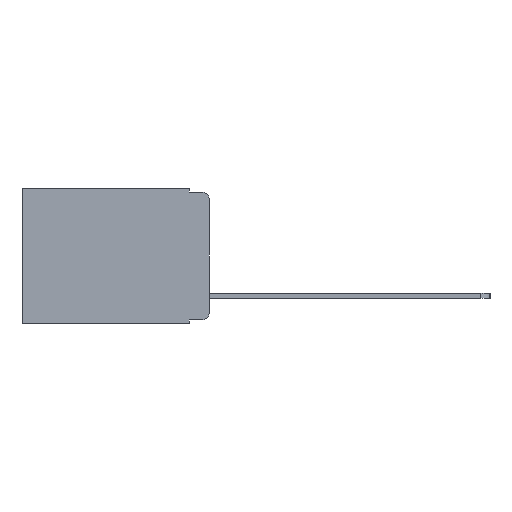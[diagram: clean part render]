
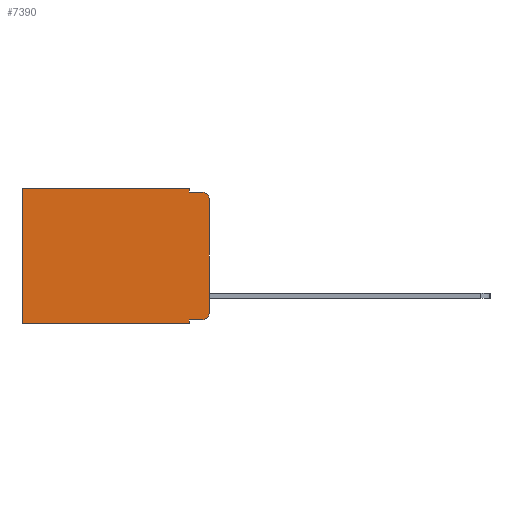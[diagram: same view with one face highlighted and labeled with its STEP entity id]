
A CAD part, left-side view. The second image highlights one B-rep face of the part: STEP entity #7390.
In plain terms, the highlighted planar face has unit normal (-1, 0, 0).
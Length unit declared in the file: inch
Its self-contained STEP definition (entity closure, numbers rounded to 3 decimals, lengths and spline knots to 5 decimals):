
#24 = ORIENTED_EDGE ( 'NONE', *, *, #18205, .T. ) ;
#71 = VERTEX_POINT ( 'NONE', #19708 ) ;
#117 = CIRCLE ( 'NONE', #6766, 0.02 ) ;
#460 = EDGE_CURVE ( 'NONE', #71, #18837, #117, .T. ) ;
#500 = LINE ( 'NONE', #4040, #9219 ) ;
#677 = CARTESIAN_POINT ( 'NONE',  ( 0.298, 0.051, 0. ) ) ;
#769 = VERTEX_POINT ( 'NONE', #20337 ) ;
#776 = CARTESIAN_POINT ( 'NONE',  ( 0.298, 0.473, -0.343 ) ) ;
#1267 = LINE ( 'NONE', #16969, #16571 ) ;
#2077 = CARTESIAN_POINT ( 'NONE',  ( 0.298, 0., 0. ) ) ;
#2133 = VERTEX_POINT ( 'NONE', #9284 ) ;
#2255 = DIRECTION ( 'NONE',  ( 0., 1., 0. ) ) ;
#3611 = CARTESIAN_POINT ( 'NONE',  ( 0.298, 0.051, -0.333 ) ) ;
#3651 = DIRECTION ( 'NONE',  ( -1., 0., 0. ) ) ;
#3672 = DIRECTION ( 'NONE',  ( -1., 0., 0. ) ) ;
#3941 = DIRECTION ( 'NONE',  ( 0., 0., -1. ) ) ;
#4040 = CARTESIAN_POINT ( 'NONE',  ( 0.298, 0., 0. ) ) ;
#4323 = ORIENTED_EDGE ( 'NONE', *, *, #22703, .T. ) ;
#4649 = ORIENTED_EDGE ( 'NONE', *, *, #11344, .F. ) ;
#5139 = PLANE ( 'NONE',  #22018 ) ;
#5387 = CARTESIAN_POINT ( 'NONE',  ( 0.298, 0.02, -0.313 ) ) ;
#5954 = DIRECTION ( 'NONE',  ( 0., -1., 0. ) ) ;
#6156 = LINE ( 'NONE', #10560, #6751 ) ;
#6223 = DIRECTION ( 'NONE',  ( 0., 0., -1. ) ) ;
#6246 = CARTESIAN_POINT ( 'NONE',  ( 0.298, 0., -0.313 ) ) ;
#6301 = LINE ( 'NONE', #8245, #11258 ) ;
#6751 = VECTOR ( 'NONE', #8712, 39.37008 ) ;
#6766 = AXIS2_PLACEMENT_3D ( 'NONE', #5387, #3672, #16507 ) ;
#6911 = ORIENTED_EDGE ( 'NONE', *, *, #20519, .F. ) ;
#7390 = ADVANCED_FACE ( 'NONE', ( #11351 ), #5139, .F. ) ;
#7611 = DIRECTION ( 'NONE',  ( 0., 0., -1. ) ) ;
#8245 = CARTESIAN_POINT ( 'NONE',  ( 0.298, 0.051, -0.01 ) ) ;
#8407 = VECTOR ( 'NONE', #8502, 39.37008 ) ;
#8502 = DIRECTION ( 'NONE',  ( 0., 0., -1. ) ) ;
#8712 = DIRECTION ( 'NONE',  ( 0., 1., 0. ) ) ;
#9081 = EDGE_CURVE ( 'NONE', #20015, #11034, #13293, .T. ) ;
#9219 = VECTOR ( 'NONE', #2255, 39.37008 ) ;
#9284 = CARTESIAN_POINT ( 'NONE',  ( 0.298, 0., -0.03 ) ) ;
#9532 = CARTESIAN_POINT ( 'NONE',  ( 0.298, 0.051, 0. ) ) ;
#10082 = VERTEX_POINT ( 'NONE', #18763 ) ;
#10102 = EDGE_CURVE ( 'NONE', #20015, #769, #500, .T. ) ;
#10287 = EDGE_LOOP ( 'NONE', ( #6911, #10393, #18681, #12419, #14443, #4323, #17871, #4649, #24, #16897 ) ) ;
#10393 = ORIENTED_EDGE ( 'NONE', *, *, #18570, .T. ) ;
#10560 = CARTESIAN_POINT ( 'NONE',  ( 0.298, 0., -0.343 ) ) ;
#11034 = VERTEX_POINT ( 'NONE', #21726 ) ;
#11258 = VECTOR ( 'NONE', #22795, 39.37008 ) ;
#11344 = EDGE_CURVE ( 'NONE', #16701, #14456, #16720, .T. ) ;
#11351 = FACE_OUTER_BOUND ( 'NONE', #10287, .T. ) ;
#11546 = LINE ( 'NONE', #16743, #20658 ) ;
#12079 = VERTEX_POINT ( 'NONE', #776 ) ;
#12223 = LINE ( 'NONE', #17232, #21868 ) ;
#12419 = ORIENTED_EDGE ( 'NONE', *, *, #9081, .F. ) ;
#13293 = LINE ( 'NONE', #17625, #8407 ) ;
#13636 = DIRECTION ( 'NONE',  ( 0., 0., -1. ) ) ;
#14017 = AXIS2_PLACEMENT_3D ( 'NONE', #14731, #3651, #16563 ) ;
#14443 = ORIENTED_EDGE ( 'NONE', *, *, #10102, .T. ) ;
#14456 = VERTEX_POINT ( 'NONE', #22624 ) ;
#14731 = CARTESIAN_POINT ( 'NONE',  ( 0.298, 0.02, -0.03 ) ) ;
#15016 = DIRECTION ( 'NONE',  ( 1., 0., 0. ) ) ;
#15937 = EDGE_CURVE ( 'NONE', #14456, #12079, #6156, .T. ) ;
#16507 = DIRECTION ( 'NONE',  ( 0., 0., -1. ) ) ;
#16563 = DIRECTION ( 'NONE',  ( 0., 0., -1. ) ) ;
#16571 = VECTOR ( 'NONE', #5954, 39.37008 ) ;
#16701 = VERTEX_POINT ( 'NONE', #3611 ) ;
#16720 = LINE ( 'NONE', #677, #22100 ) ;
#16743 = CARTESIAN_POINT ( 'NONE',  ( 0.298, 0.473, 0. ) ) ;
#16897 = ORIENTED_EDGE ( 'NONE', *, *, #460, .T. ) ;
#16969 = CARTESIAN_POINT ( 'NONE',  ( 0.298, 0.051, -0.333 ) ) ;
#17232 = CARTESIAN_POINT ( 'NONE',  ( 0.298, 0., 0. ) ) ;
#17625 = CARTESIAN_POINT ( 'NONE',  ( 0.298, 0.051, 0. ) ) ;
#17871 = ORIENTED_EDGE ( 'NONE', *, *, #15937, .F. ) ;
#18205 = EDGE_CURVE ( 'NONE', #16701, #71, #1267, .T. ) ;
#18570 = EDGE_CURVE ( 'NONE', #2133, #10082, #21925, .T. ) ;
#18681 = ORIENTED_EDGE ( 'NONE', *, *, #22924, .F. ) ;
#18763 = CARTESIAN_POINT ( 'NONE',  ( 0.298, 0.02, -0.01 ) ) ;
#18837 = VERTEX_POINT ( 'NONE', #6246 ) ;
#19708 = CARTESIAN_POINT ( 'NONE',  ( 0.298, 0.02, -0.333 ) ) ;
#20015 = VERTEX_POINT ( 'NONE', #9532 ) ;
#20337 = CARTESIAN_POINT ( 'NONE',  ( 0.298, 0.473, 0. ) ) ;
#20519 = EDGE_CURVE ( 'NONE', #2133, #18837, #12223, .T. ) ;
#20658 = VECTOR ( 'NONE', #7611, 39.37008 ) ;
#21726 = CARTESIAN_POINT ( 'NONE',  ( 0.298, 0.051, -0.01 ) ) ;
#21868 = VECTOR ( 'NONE', #6223, 39.37008 ) ;
#21925 = CIRCLE ( 'NONE', #14017, 0.02 ) ;
#22018 = AXIS2_PLACEMENT_3D ( 'NONE', #2077, #15016, #3941 ) ;
#22100 = VECTOR ( 'NONE', #13636, 39.37008 ) ;
#22624 = CARTESIAN_POINT ( 'NONE',  ( 0.298, 0.051, -0.343 ) ) ;
#22703 = EDGE_CURVE ( 'NONE', #769, #12079, #11546, .T. ) ;
#22795 = DIRECTION ( 'NONE',  ( 0., -1., 0. ) ) ;
#22924 = EDGE_CURVE ( 'NONE', #11034, #10082, #6301, .T. ) ;
